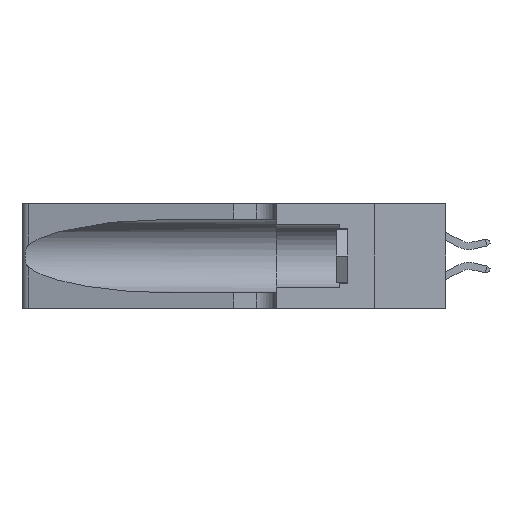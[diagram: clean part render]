
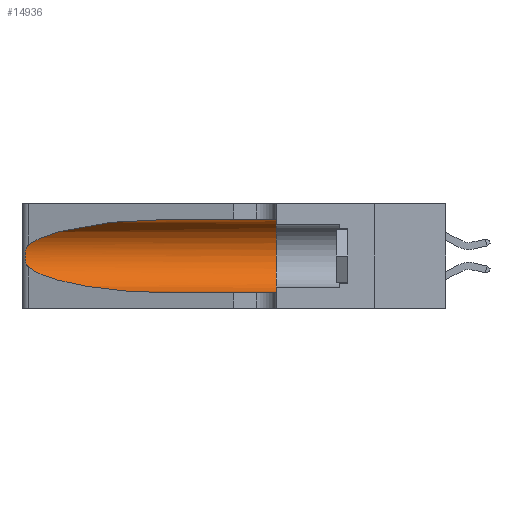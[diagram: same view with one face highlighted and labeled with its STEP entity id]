
A CAD part, left-side view. The second image highlights one B-rep face of the part: STEP entity #14936.
In plain terms, the highlighted cylindrical face has radius 3.308 mm (diameter 6.617 mm), a partial arc.
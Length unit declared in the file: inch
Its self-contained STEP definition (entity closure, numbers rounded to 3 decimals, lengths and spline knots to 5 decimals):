
#523 = VERTEX_POINT ( 'NONE', #28013 ) ;
#1004 = ORIENTED_EDGE ( 'NONE', *, *, #21509, .T. ) ;
#1957 = CARTESIAN_POINT ( 'NONE',  ( 0.25487, 1.22718, 0.14631 ) ) ;
#2262 = DIRECTION ( 'NONE',  ( 0., 0., 1. ) ) ;
#2270 = CARTESIAN_POINT ( 'NONE',  ( 0.1305, 0.35, 0.05475 ) ) ;
#2443 = B_SPLINE_CURVE_WITH_KNOTS ( 'NONE', 3,
 ( #13301, #10671, #15922, #34037, #18494, #2681, #21108, #5393, #23737, #8131, #26329, #10790, #28989, #13424 ),
 .UNSPECIFIED., .F., .F.,
 ( 4, 2, 2, 2, 2, 2, 4 ),
 ( 0., 0.00027, 0.00053, 0.00107, 0.0016, 0.00187, 0.00214 ),
 .UNSPECIFIED. ) ;
#2681 = CARTESIAN_POINT ( 'NONE',  ( 0.26018, 1.23835, 0.19895 ) ) ;
#2738 = ORIENTED_EDGE ( 'NONE', *, *, #24831, .F. ) ;
#3585 = ORIENTED_EDGE ( 'NONE', *, *, #23899, .F. ) ;
#4385 = EDGE_CURVE ( 'NONE', #26479, #4449, #5050, .T. ) ;
#4449 = VERTEX_POINT ( 'NONE', #33392 ) ;
#4687 = CARTESIAN_POINT ( 'NONE',  ( 0.18966, 0.96281, 0.05475 ) ) ;
#4780 = DIRECTION ( 'NONE',  ( 0., -1., 0. ) ) ;
#5050 =( BOUNDED_CURVE ( )  B_SPLINE_CURVE ( 3, ( #27993, #25369, #9783, #12425 ),
 .UNSPECIFIED., .F., .F. ) 
 B_SPLINE_CURVE_WITH_KNOTS ( ( 4, 4 ),
 ( 1.5708, 2.84003 ),
 .UNSPECIFIED. ) 
 CURVE ( )  GEOMETRIC_REPRESENTATION_ITEM ( )  RATIONAL_B_SPLINE_CURVE ( ( 1., 0.87, 0.87, 1. ) ) 
 REPRESENTATION_ITEM ( '' )  );
#5393 = CARTESIAN_POINT ( 'NONE',  ( 0.26075, 1.23896, 0.178 ) ) ;
#5778 = VERTEX_POINT ( 'NONE', #2270 ) ;
#6672 = CARTESIAN_POINT ( 'NONE',  ( 0.1305, 0.72297, 0.31525 ) ) ;
#7731 = CARTESIAN_POINT ( 'NONE',  ( 0.1305, 1.61858, 0.185 ) ) ;
#7912 = CARTESIAN_POINT ( 'NONE',  ( 0.1305, 1.61858, 0.05475 ) ) ;
#7959 = CARTESIAN_POINT ( 'NONE',  ( 0.1305, 0.72297, 0.05475 ) ) ;
#8131 = CARTESIAN_POINT ( 'NONE',  ( 0.25856, 1.23593, 0.16098 ) ) ;
#8388 = EDGE_CURVE ( 'NONE', #523, #11230, #26878, .T. ) ;
#9783 = CARTESIAN_POINT ( 'NONE',  ( 0.2373, 1.15595, 0.28018 ) ) ;
#9940 = EDGE_CURVE ( 'NONE', #11230, #5778, #10356, .T. ) ;
#10356 = LINE ( 'NONE', #7912, #30315 ) ;
#10386 = DIRECTION ( 'NONE',  ( 0., -1., 0. ) ) ;
#10671 = CARTESIAN_POINT ( 'NONE',  ( 0.25555, 1.22994, 0.2215 ) ) ;
#10790 = CARTESIAN_POINT ( 'NONE',  ( 0.25639, 1.23186, 0.15144 ) ) ;
#11230 = VERTEX_POINT ( 'NONE', #7959 ) ;
#12425 = CARTESIAN_POINT ( 'NONE',  ( 0.25487, 1.22718, 0.22369 ) ) ;
#13248 = EDGE_LOOP ( 'NONE', ( #21282, #1004, #29044, #16034, #2738, #3585 ) ) ;
#13301 = CARTESIAN_POINT ( 'NONE',  ( 0.25487, 1.22718, 0.22369 ) ) ;
#13424 = CARTESIAN_POINT ( 'NONE',  ( 0.25487, 1.22718, 0.14631 ) ) ;
#13434 = VECTOR ( 'NONE', #4780, 39.37008 ) ;
#14936 = ADVANCED_FACE ( 'NONE', ( #33109 ), #32296, .F. ) ;
#14963 = CARTESIAN_POINT ( 'NONE',  ( 0.1305, 0.35, 0.31525 ) ) ;
#15922 = CARTESIAN_POINT ( 'NONE',  ( 0.25639, 1.23184, 0.21858 ) ) ;
#16034 = ORIENTED_EDGE ( 'NONE', *, *, #9940, .T. ) ;
#17850 = CARTESIAN_POINT ( 'NONE',  ( 0.2373, 1.15595, 0.08982 ) ) ;
#18115 = DIRECTION ( 'NONE',  ( 0., 1., 0. ) ) ;
#18494 = CARTESIAN_POINT ( 'NONE',  ( 0.25854, 1.2359, 0.20912 ) ) ;
#19492 = LINE ( 'NONE', #28385, #13434 ) ;
#21108 = CARTESIAN_POINT ( 'NONE',  ( 0.26075, 1.23896, 0.19203 ) ) ;
#21282 = ORIENTED_EDGE ( 'NONE', *, *, #4385, .T. ) ;
#21509 = EDGE_CURVE ( 'NONE', #4449, #523, #2443, .T. ) ;
#23068 = CARTESIAN_POINT ( 'NONE',  ( 0.1305, 0.72297, 0.05475 ) ) ;
#23737 = CARTESIAN_POINT ( 'NONE',  ( 0.26017, 1.23833, 0.17102 ) ) ;
#23899 = EDGE_CURVE ( 'NONE', #26479, #30520, #19492, .T. ) ;
#24831 = EDGE_CURVE ( 'NONE', #30520, #5778, #25989, .T. ) ;
#25369 = CARTESIAN_POINT ( 'NONE',  ( 0.18966, 0.96281, 0.31525 ) ) ;
#25719 = AXIS2_PLACEMENT_3D ( 'NONE', #7731, #10386, #28601 ) ;
#25989 = CIRCLE ( 'NONE', #26150, 0.13025 ) ;
#26150 = AXIS2_PLACEMENT_3D ( 'NONE', #33649, #18115, #2262 ) ;
#26329 = CARTESIAN_POINT ( 'NONE',  ( 0.25789, 1.23486, 0.15765 ) ) ;
#26479 = VERTEX_POINT ( 'NONE', #6672 ) ;
#26878 =( BOUNDED_CURVE ( )  B_SPLINE_CURVE ( 3, ( #1957, #17850, #4687, #23068 ),
 .UNSPECIFIED., .F., .F. ) 
 B_SPLINE_CURVE_WITH_KNOTS ( ( 4, 4 ),
 ( 3.44316, 4.71239 ),
 .UNSPECIFIED. ) 
 CURVE ( )  GEOMETRIC_REPRESENTATION_ITEM ( )  RATIONAL_B_SPLINE_CURVE ( ( 1., 0.87, 0.87, 1. ) ) 
 REPRESENTATION_ITEM ( '' )  );
#27993 = CARTESIAN_POINT ( 'NONE',  ( 0.1305, 0.72297, 0.31525 ) ) ;
#28013 = CARTESIAN_POINT ( 'NONE',  ( 0.25487, 1.22718, 0.14631 ) ) ;
#28385 = CARTESIAN_POINT ( 'NONE',  ( 0.1305, 1.61858, 0.31525 ) ) ;
#28601 = DIRECTION ( 'NONE',  ( 0., 0., -1. ) ) ;
#28989 = CARTESIAN_POINT ( 'NONE',  ( 0.25555, 1.22993, 0.14849 ) ) ;
#29044 = ORIENTED_EDGE ( 'NONE', *, *, #8388, .T. ) ;
#30315 = VECTOR ( 'NONE', #31347, 39.37008 ) ;
#30520 = VERTEX_POINT ( 'NONE', #14963 ) ;
#31347 = DIRECTION ( 'NONE',  ( 0., -1., 0. ) ) ;
#32296 = CYLINDRICAL_SURFACE ( 'NONE', #25719, 0.13025 ) ;
#33109 = FACE_OUTER_BOUND ( 'NONE', #13248, .T. ) ;
#33392 = CARTESIAN_POINT ( 'NONE',  ( 0.25487, 1.22718, 0.22369 ) ) ;
#33649 = CARTESIAN_POINT ( 'NONE',  ( 0.1305, 0.35, 0.185 ) ) ;
#34037 = CARTESIAN_POINT ( 'NONE',  ( 0.25787, 1.23484, 0.2124 ) ) ;
